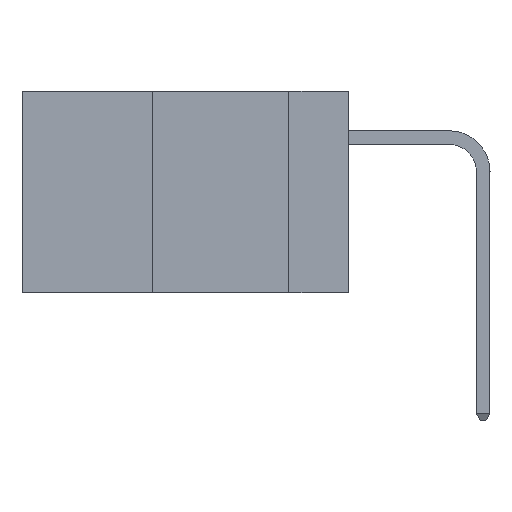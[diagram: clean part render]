
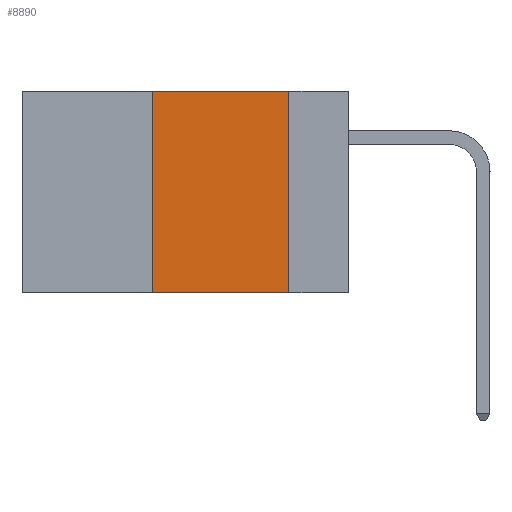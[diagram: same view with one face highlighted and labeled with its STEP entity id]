
A CAD part, left-side view. The second image highlights one B-rep face of the part: STEP entity #8890.
In plain terms, the highlighted planar face has unit normal (-1, 0, 0).
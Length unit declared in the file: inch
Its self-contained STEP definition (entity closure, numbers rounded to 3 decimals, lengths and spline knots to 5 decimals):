
#744 = VECTOR ( 'NONE', #5663, 39.37008 ) ;
#840 = CARTESIAN_POINT ( 'NONE',  ( 0., 0.11, 0. ) ) ;
#911 = LINE ( 'NONE', #15664, #4462 ) ;
#1046 = VERTEX_POINT ( 'NONE', #14018 ) ;
#1541 = CARTESIAN_POINT ( 'NONE',  ( 0., 0.11, -0.37 ) ) ;
#2114 = CARTESIAN_POINT ( 'NONE',  ( 0., 0.36, 0. ) ) ;
#2560 = ORIENTED_EDGE ( 'NONE', *, *, #8102, .F. ) ;
#2697 = VERTEX_POINT ( 'NONE', #2114 ) ;
#3231 = LINE ( 'NONE', #14637, #18128 ) ;
#3554 = ORIENTED_EDGE ( 'NONE', *, *, #9538, .F. ) ;
#3831 = CARTESIAN_POINT ( 'NONE',  ( 0., 0.6, 0. ) ) ;
#4091 = VERTEX_POINT ( 'NONE', #13883 ) ;
#4366 = ORIENTED_EDGE ( 'NONE', *, *, #16359, .F. ) ;
#4462 = VECTOR ( 'NONE', #7123, 39.37008 ) ;
#4989 = LINE ( 'NONE', #14467, #8982 ) ;
#5363 = PLANE ( 'NONE',  #8869 ) ;
#5663 = DIRECTION ( 'NONE',  ( 0., 0., -1. ) ) ;
#5849 = DIRECTION ( 'NONE',  ( 0., 0., 1. ) ) ;
#6778 = EDGE_LOOP ( 'NONE', ( #2560, #3554, #4366, #13336 ) ) ;
#6883 = DIRECTION ( 'NONE',  ( 0., 0., -1. ) ) ;
#7123 = DIRECTION ( 'NONE',  ( 0., -1., 0. ) ) ;
#8102 = EDGE_CURVE ( 'NONE', #4091, #14812, #12941, .T. ) ;
#8869 = AXIS2_PLACEMENT_3D ( 'NONE', #3831, #15448, #6883 ) ;
#8890 = ADVANCED_FACE ( 'NONE', ( #11579 ), #5363, .F. ) ;
#8982 = VECTOR ( 'NONE', #5849, 39.37008 ) ;
#9538 = EDGE_CURVE ( 'NONE', #2697, #4091, #911, .T. ) ;
#11579 = FACE_OUTER_BOUND ( 'NONE', #6778, .T. ) ;
#12941 = LINE ( 'NONE', #840, #744 ) ;
#13336 = ORIENTED_EDGE ( 'NONE', *, *, #18314, .T. ) ;
#13883 = CARTESIAN_POINT ( 'NONE',  ( 0., 0.11, 0. ) ) ;
#14018 = CARTESIAN_POINT ( 'NONE',  ( 0., 0.36, -0.37 ) ) ;
#14467 = CARTESIAN_POINT ( 'NONE',  ( 0., 0.36, 0. ) ) ;
#14637 = CARTESIAN_POINT ( 'NONE',  ( 0., 0.6, -0.37 ) ) ;
#14812 = VERTEX_POINT ( 'NONE', #1541 ) ;
#15448 = DIRECTION ( 'NONE',  ( 1., 0., 0. ) ) ;
#15664 = CARTESIAN_POINT ( 'NONE',  ( 0., 0.6, 0. ) ) ;
#16359 = EDGE_CURVE ( 'NONE', #1046, #2697, #4989, .T. ) ;
#17459 = DIRECTION ( 'NONE',  ( 0., -1., 0. ) ) ;
#18128 = VECTOR ( 'NONE', #17459, 39.37008 ) ;
#18314 = EDGE_CURVE ( 'NONE', #1046, #14812, #3231, .T. ) ;
